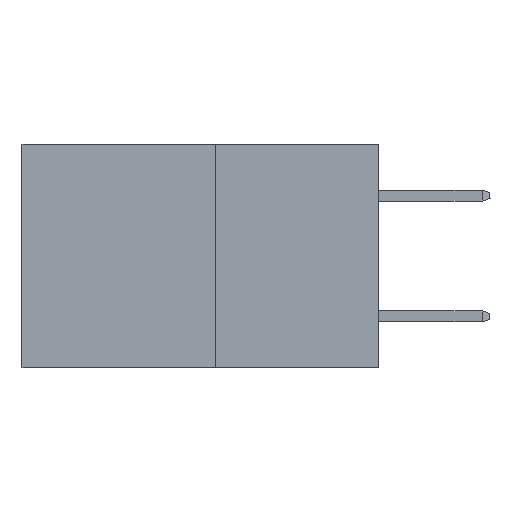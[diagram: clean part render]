
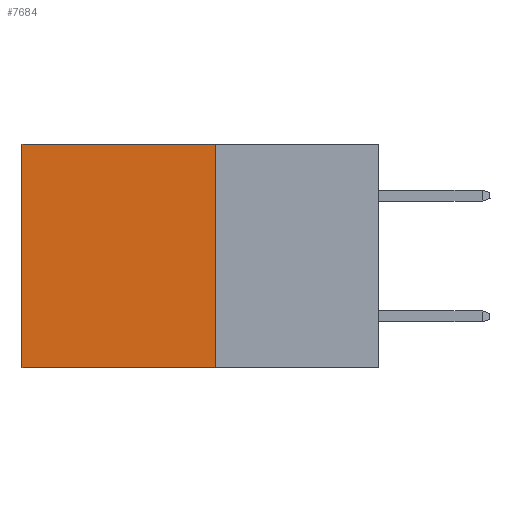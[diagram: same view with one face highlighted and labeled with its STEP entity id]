
A CAD part, left-side view. The second image highlights one B-rep face of the part: STEP entity #7684.
In plain terms, the highlighted planar face has unit normal (-1, 0, 0).
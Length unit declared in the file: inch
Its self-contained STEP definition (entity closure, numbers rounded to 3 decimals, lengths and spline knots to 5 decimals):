
#604 = ORIENTED_EDGE ( 'NONE', *, *, #1355, .T. ) ;
#908 = DIRECTION ( 'NONE',  ( 0., 0., -1. ) ) ;
#944 = CARTESIAN_POINT ( 'NONE',  ( 0.277, 0.27, -0.37 ) ) ;
#1355 = EDGE_CURVE ( 'NONE', #1893, #11098, #15308, .T. ) ;
#1679 = EDGE_LOOP ( 'NONE', ( #12472, #3424, #12857, #604 ) ) ;
#1877 = VERTEX_POINT ( 'NONE', #8423 ) ;
#1893 = VERTEX_POINT ( 'NONE', #6146 ) ;
#2263 = LINE ( 'NONE', #944, #5136 ) ;
#2341 = LINE ( 'NONE', #4631, #14552 ) ;
#3118 = VECTOR ( 'NONE', #5325, 39.37008 ) ;
#3424 = ORIENTED_EDGE ( 'NONE', *, *, #6001, .F. ) ;
#3554 = EDGE_CURVE ( 'NONE', #11098, #10366, #14319, .T. ) ;
#3801 = CARTESIAN_POINT ( 'NONE',  ( 0.277, 0.27, 0. ) ) ;
#4350 = CARTESIAN_POINT ( 'NONE',  ( 0.277, 0.59, 0. ) ) ;
#4499 = DIRECTION ( 'NONE',  ( 0., 1., 0. ) ) ;
#4631 = CARTESIAN_POINT ( 'NONE',  ( 0.277, 0.27, -0.37 ) ) ;
#5136 = VECTOR ( 'NONE', #908, 39.37008 ) ;
#5153 = FACE_OUTER_BOUND ( 'NONE', #1679, .T. ) ;
#5263 = DIRECTION ( 'NONE',  ( 0., 0., -1. ) ) ;
#5278 = CARTESIAN_POINT ( 'NONE',  ( 0.277, 0.59, -0.37 ) ) ;
#5284 = DIRECTION ( 'NONE',  ( 1., 0., 0. ) ) ;
#5299 = PLANE ( 'NONE',  #6377 ) ;
#5305 = CARTESIAN_POINT ( 'NONE',  ( 0.277, 0.27, -0.37 ) ) ;
#5325 = DIRECTION ( 'NONE',  ( 0., 1., 0. ) ) ;
#5362 = VECTOR ( 'NONE', #5589, 39.37008 ) ;
#5589 = DIRECTION ( 'NONE',  ( 0., 0., -1. ) ) ;
#6001 = EDGE_CURVE ( 'NONE', #1877, #10366, #2341, .T. ) ;
#6146 = CARTESIAN_POINT ( 'NONE',  ( 0.277, 0.27, 0. ) ) ;
#6377 = AXIS2_PLACEMENT_3D ( 'NONE', #5305, #5284, #5263 ) ;
#7684 = ADVANCED_FACE ( 'NONE', ( #5153 ), #5299, .F. ) ;
#8083 = EDGE_CURVE ( 'NONE', #1893, #1877, #2263, .T. ) ;
#8423 = CARTESIAN_POINT ( 'NONE',  ( 0.277, 0.27, -0.37 ) ) ;
#10366 = VERTEX_POINT ( 'NONE', #11190 ) ;
#11098 = VERTEX_POINT ( 'NONE', #4350 ) ;
#11190 = CARTESIAN_POINT ( 'NONE',  ( 0.277, 0.59, -0.37 ) ) ;
#12472 = ORIENTED_EDGE ( 'NONE', *, *, #3554, .T. ) ;
#12857 = ORIENTED_EDGE ( 'NONE', *, *, #8083, .F. ) ;
#14319 = LINE ( 'NONE', #5278, #5362 ) ;
#14552 = VECTOR ( 'NONE', #4499, 39.37008 ) ;
#15308 = LINE ( 'NONE', #3801, #3118 ) ;
